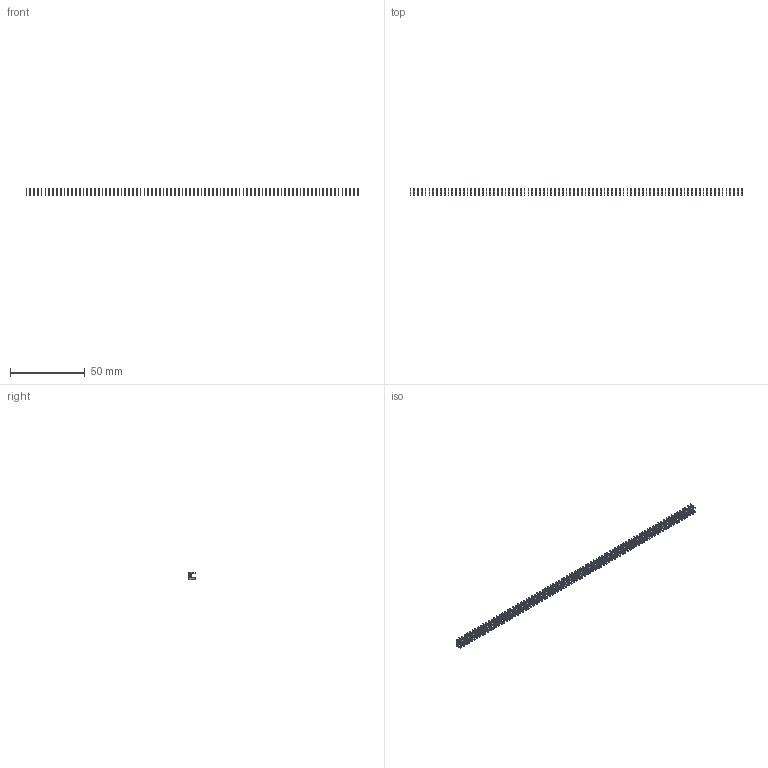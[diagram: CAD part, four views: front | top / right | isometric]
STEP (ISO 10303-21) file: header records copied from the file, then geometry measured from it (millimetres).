
FILE_DESCRIPTION (( 'STEP AP203' ), '1' );
FILE_NAME ('105-088-208-100.STEP', '2020-04-08T01:11:40', ( '' ), ( '' ), 'SwSTEP 2.0', 'SolidWorks 2016', '' );
FILE_SCHEMA (( 'CONFIG_CONTROL_DESIGN' ));
Length unit declared in the file: inch
Products named in the file (2): 100-290-001_100-290-208; 105-088-208-100
Assembly tree (88 placements, depth 2):
  105-088-208-100
    100-290-001_100-290-208  x88
Bounding box: 221.49 x 4.83 x 5.17 mm (x, y, z)
Volume: 605.5 mm3; surface area: 3739.7 mm2
Topology: 88 solids, 88 shells, 2200 faces, 6072 edges, 4048 vertices
Faces by surface type: plane 1936, cylinder 264
Entity records: 3773 total; most frequent: DIRECTION 307, CARTESIAN_POINT 231, LOCAL_TIME 186, COORDINATED_UNIVERSAL_TIME_OFFSET 186, CALENDAR_DATE 186, DATE_AND_TIME 186, ORIENTED_EDGE 138, AXIS2_PLACEMENT_3D 122
